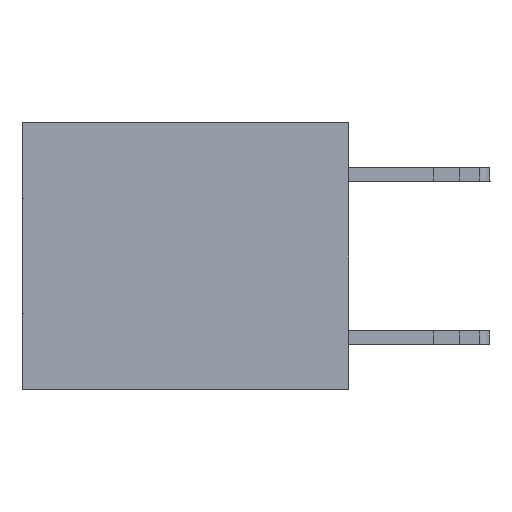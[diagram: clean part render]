
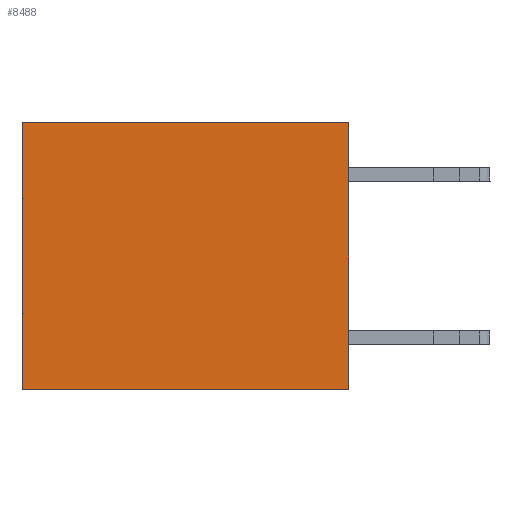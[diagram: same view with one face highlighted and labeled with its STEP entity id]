
A CAD part, left-side view. The second image highlights one B-rep face of the part: STEP entity #8488.
In plain terms, the highlighted planar face has unit normal (-1, 0, 0).
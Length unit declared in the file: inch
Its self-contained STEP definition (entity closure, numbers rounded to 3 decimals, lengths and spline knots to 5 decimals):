
#70 = ORIENTED_EDGE ( 'NONE', *, *, #21252, .T. ) ;
#639 = CARTESIAN_POINT ( 'NONE',  ( 0.3165, 0.6, -0.49 ) ) ;
#717 = ORIENTED_EDGE ( 'NONE', *, *, #19999, .F. ) ;
#828 = VERTEX_POINT ( 'NONE', #18199 ) ;
#1177 = CARTESIAN_POINT ( 'NONE',  ( 0.3165, 0., -0.49 ) ) ;
#2116 = VERTEX_POINT ( 'NONE', #23211 ) ;
#2594 = EDGE_LOOP ( 'NONE', ( #22008, #30577, #717, #70 ) ) ;
#3332 = DIRECTION ( 'NONE',  ( 0., 0., -1. ) ) ;
#4339 = VECTOR ( 'NONE', #18995, 39.37008 ) ;
#7581 = CARTESIAN_POINT ( 'NONE',  ( 0.3165, 0.6, -0.49 ) ) ;
#8488 = ADVANCED_FACE ( 'NONE', ( #10400 ), #21579, .F. ) ;
#10400 = FACE_OUTER_BOUND ( 'NONE', #2594, .T. ) ;
#10415 = VECTOR ( 'NONE', #17418, 39.37008 ) ;
#12139 = LINE ( 'NONE', #639, #4339 ) ;
#12479 = CARTESIAN_POINT ( 'NONE',  ( 0.3165, 0., 0. ) ) ;
#14576 = DIRECTION ( 'NONE',  ( 1., 0., 0. ) ) ;
#14676 = CARTESIAN_POINT ( 'NONE',  ( 0.3165, 0., -0.49 ) ) ;
#16591 = VECTOR ( 'NONE', #3332, 39.37008 ) ;
#17418 = DIRECTION ( 'NONE',  ( 0., 1., 0. ) ) ;
#18199 = CARTESIAN_POINT ( 'NONE',  ( 0.3165, 0.6, 0. ) ) ;
#18972 = EDGE_CURVE ( 'NONE', #828, #31448, #12139, .T. ) ;
#18995 = DIRECTION ( 'NONE',  ( 0., 0., -1. ) ) ;
#19995 = VECTOR ( 'NONE', #20476, 39.37008 ) ;
#19999 = EDGE_CURVE ( 'NONE', #2116, #20772, #30501, .T. ) ;
#20476 = DIRECTION ( 'NONE',  ( 0., 1., 0. ) ) ;
#20772 = VERTEX_POINT ( 'NONE', #28971 ) ;
#21252 = EDGE_CURVE ( 'NONE', #2116, #828, #21635, .T. ) ;
#21579 = PLANE ( 'NONE',  #25531 ) ;
#21635 = LINE ( 'NONE', #12479, #19995 ) ;
#22008 = ORIENTED_EDGE ( 'NONE', *, *, #18972, .T. ) ;
#22141 = DIRECTION ( 'NONE',  ( 0., 0., -1. ) ) ;
#23211 = CARTESIAN_POINT ( 'NONE',  ( 0.3165, 0., 0. ) ) ;
#24132 = CARTESIAN_POINT ( 'NONE',  ( 0.3165, 0., -0.49 ) ) ;
#25531 = AXIS2_PLACEMENT_3D ( 'NONE', #1177, #14576, #22141 ) ;
#26488 = EDGE_CURVE ( 'NONE', #20772, #31448, #27966, .T. ) ;
#27966 = LINE ( 'NONE', #14676, #10415 ) ;
#28971 = CARTESIAN_POINT ( 'NONE',  ( 0.3165, 0., -0.49 ) ) ;
#30501 = LINE ( 'NONE', #24132, #16591 ) ;
#30577 = ORIENTED_EDGE ( 'NONE', *, *, #26488, .F. ) ;
#31448 = VERTEX_POINT ( 'NONE', #7581 ) ;
